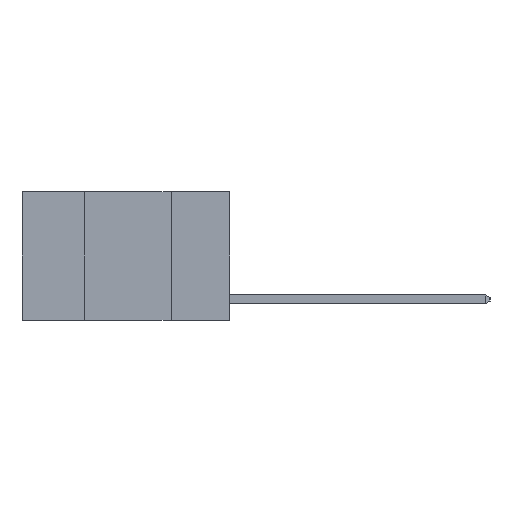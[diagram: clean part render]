
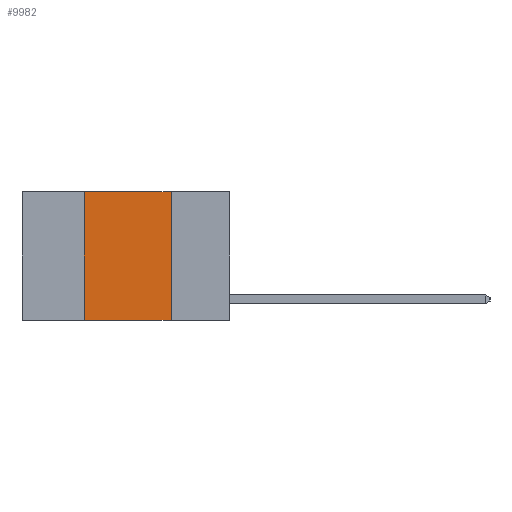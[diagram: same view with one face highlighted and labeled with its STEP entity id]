
A CAD part, left-side view. The second image highlights one B-rep face of the part: STEP entity #9982.
In plain terms, the highlighted planar face has unit normal (-1, 0, 0).
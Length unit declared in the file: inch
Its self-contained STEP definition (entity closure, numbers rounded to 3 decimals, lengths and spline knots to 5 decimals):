
#201 = AXIS2_PLACEMENT_3D ( 'NONE', #6729, #2364, #8516 ) ;
#663 = CARTESIAN_POINT ( 'NONE',  ( 0., 0.42, 0. ) ) ;
#669 = DIRECTION ( 'NONE',  ( 0., -1., 0. ) ) ;
#706 = DIRECTION ( 'NONE',  ( 0., 0., 1. ) ) ;
#919 = VERTEX_POINT ( 'NONE', #9496 ) ;
#1081 = VERTEX_POINT ( 'NONE', #2030 ) ;
#1163 = DIRECTION ( 'NONE',  ( 0., 0., -1. ) ) ;
#1363 = EDGE_CURVE ( 'NONE', #1081, #6897, #4896, .T. ) ;
#2030 = CARTESIAN_POINT ( 'NONE',  ( 0., 0.42, -0.37 ) ) ;
#2364 = DIRECTION ( 'NONE',  ( 1., 0., 0. ) ) ;
#2553 = VECTOR ( 'NONE', #706, 39.37008 ) ;
#2994 = ORIENTED_EDGE ( 'NONE', *, *, #4547, .F. ) ;
#3183 = CARTESIAN_POINT ( 'NONE',  ( 0., 0.6, 0. ) ) ;
#3263 = CARTESIAN_POINT ( 'NONE',  ( 0., 0.42, 0. ) ) ;
#3436 = ORIENTED_EDGE ( 'NONE', *, *, #1363, .F. ) ;
#3736 = EDGE_CURVE ( 'NONE', #9497, #919, #8110, .T. ) ;
#3891 = ORIENTED_EDGE ( 'NONE', *, *, #8681, .T. ) ;
#4015 = VECTOR ( 'NONE', #1163, 39.37008 ) ;
#4547 = EDGE_CURVE ( 'NONE', #6897, #9497, #8378, .T. ) ;
#4896 = LINE ( 'NONE', #663, #2553 ) ;
#4930 = LINE ( 'NONE', #11210, #7514 ) ;
#5152 = CARTESIAN_POINT ( 'NONE',  ( 0., 0.17, 0. ) ) ;
#6300 = VECTOR ( 'NONE', #9320, 39.37008 ) ;
#6729 = CARTESIAN_POINT ( 'NONE',  ( 0., 0.6, 0. ) ) ;
#6897 = VERTEX_POINT ( 'NONE', #3263 ) ;
#7303 = CARTESIAN_POINT ( 'NONE',  ( 0., 0.17, 0. ) ) ;
#7514 = VECTOR ( 'NONE', #669, 39.37008 ) ;
#8110 = LINE ( 'NONE', #7303, #4015 ) ;
#8378 = LINE ( 'NONE', #3183, #6300 ) ;
#8516 = DIRECTION ( 'NONE',  ( 0., 0., -1. ) ) ;
#8681 = EDGE_CURVE ( 'NONE', #1081, #919, #4930, .T. ) ;
#9320 = DIRECTION ( 'NONE',  ( 0., -1., 0. ) ) ;
#9369 = PLANE ( 'NONE',  #201 ) ;
#9496 = CARTESIAN_POINT ( 'NONE',  ( 0., 0.17, -0.37 ) ) ;
#9497 = VERTEX_POINT ( 'NONE', #5152 ) ;
#9982 = ADVANCED_FACE ( 'NONE', ( #10099 ), #9369, .F. ) ;
#10099 = FACE_OUTER_BOUND ( 'NONE', #10691, .T. ) ;
#10691 = EDGE_LOOP ( 'NONE', ( #10980, #2994, #3436, #3891 ) ) ;
#10980 = ORIENTED_EDGE ( 'NONE', *, *, #3736, .F. ) ;
#11210 = CARTESIAN_POINT ( 'NONE',  ( 0., 0.6, -0.37 ) ) ;
